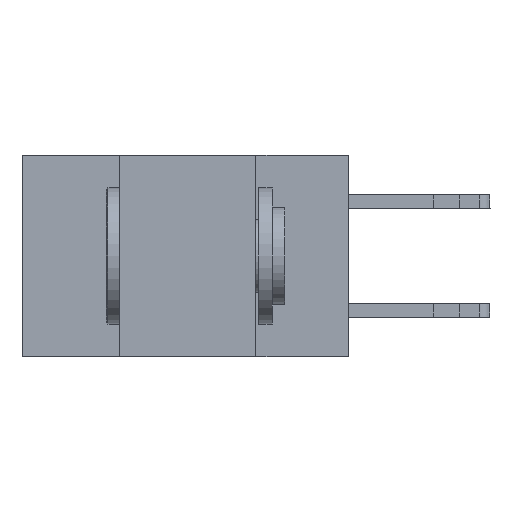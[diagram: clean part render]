
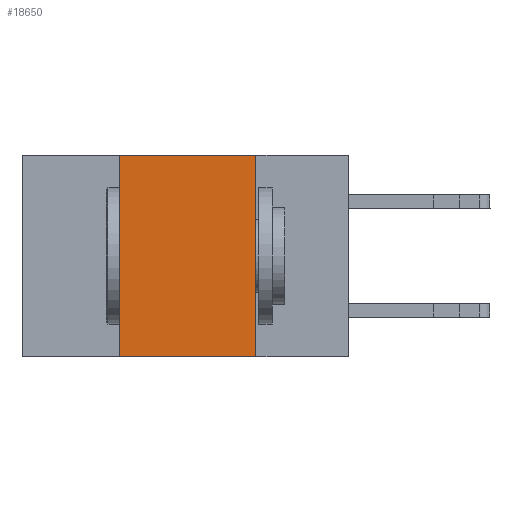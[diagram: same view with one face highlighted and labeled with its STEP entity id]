
A CAD part, left-side view. The second image highlights one B-rep face of the part: STEP entity #18650.
In plain terms, the highlighted planar face has unit normal (-1, 0, 0).
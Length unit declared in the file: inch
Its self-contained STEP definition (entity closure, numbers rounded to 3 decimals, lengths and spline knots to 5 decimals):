
#201 = DIRECTION ( 'NONE',  ( 0., 0., -1. ) ) ;
#992 = CARTESIAN_POINT ( 'NONE',  ( 0., 0.42, -0.37 ) ) ;
#1176 = VECTOR ( 'NONE', #9936, 39.37008 ) ;
#1830 = CARTESIAN_POINT ( 'NONE',  ( 0., 0.6, 0. ) ) ;
#1969 = ORIENTED_EDGE ( 'NONE', *, *, #13369, .F. ) ;
#2832 = ORIENTED_EDGE ( 'NONE', *, *, #12602, .F. ) ;
#3264 = CARTESIAN_POINT ( 'NONE',  ( 0., 0.42, -0.37 ) ) ;
#3467 = DIRECTION ( 'NONE',  ( 0., 0., 1. ) ) ;
#3543 = CARTESIAN_POINT ( 'NONE',  ( 0., 0.6, -0.37 ) ) ;
#3649 = CARTESIAN_POINT ( 'NONE',  ( 0., 0.17, -0.37 ) ) ;
#3919 = CARTESIAN_POINT ( 'NONE',  ( 0., 0.6, 0. ) ) ;
#3956 = LINE ( 'NONE', #3649, #19135 ) ;
#4370 = AXIS2_PLACEMENT_3D ( 'NONE', #1830, #17554, #201 ) ;
#5121 = CARTESIAN_POINT ( 'NONE',  ( 0., 0.42, 0. ) ) ;
#5311 = EDGE_CURVE ( 'NONE', #19190, #16157, #6122, .T. ) ;
#6012 = VERTEX_POINT ( 'NONE', #16229 ) ;
#6122 = LINE ( 'NONE', #3264, #13753 ) ;
#6465 = ORIENTED_EDGE ( 'NONE', *, *, #5311, .F. ) ;
#7009 = DIRECTION ( 'NONE',  ( 0., 0., -1. ) ) ;
#7177 = DIRECTION ( 'NONE',  ( 0., -1., 0. ) ) ;
#7364 = EDGE_CURVE ( 'NONE', #19190, #18575, #14701, .T. ) ;
#7550 = ORIENTED_EDGE ( 'NONE', *, *, #7364, .T. ) ;
#9936 = DIRECTION ( 'NONE',  ( 0., -1., 0. ) ) ;
#10732 = VECTOR ( 'NONE', #7177, 39.37008 ) ;
#12602 = EDGE_CURVE ( 'NONE', #16157, #6012, #18212, .T. ) ;
#12871 = FACE_OUTER_BOUND ( 'NONE', #12875, .T. ) ;
#12875 = EDGE_LOOP ( 'NONE', ( #1969, #2832, #6465, #7550 ) ) ;
#13369 = EDGE_CURVE ( 'NONE', #6012, #18575, #3956, .T. ) ;
#13753 = VECTOR ( 'NONE', #3467, 39.37008 ) ;
#14701 = LINE ( 'NONE', #3543, #1176 ) ;
#15831 = PLANE ( 'NONE',  #4370 ) ;
#16157 = VERTEX_POINT ( 'NONE', #5121 ) ;
#16229 = CARTESIAN_POINT ( 'NONE',  ( 0., 0.17, 0. ) ) ;
#16849 = CARTESIAN_POINT ( 'NONE',  ( 0., 0.17, -0.37 ) ) ;
#17554 = DIRECTION ( 'NONE',  ( 1., 0., 0. ) ) ;
#18212 = LINE ( 'NONE', #3919, #10732 ) ;
#18575 = VERTEX_POINT ( 'NONE', #16849 ) ;
#18650 = ADVANCED_FACE ( 'NONE', ( #12871 ), #15831, .F. ) ;
#19135 = VECTOR ( 'NONE', #7009, 39.37008 ) ;
#19190 = VERTEX_POINT ( 'NONE', #992 ) ;
